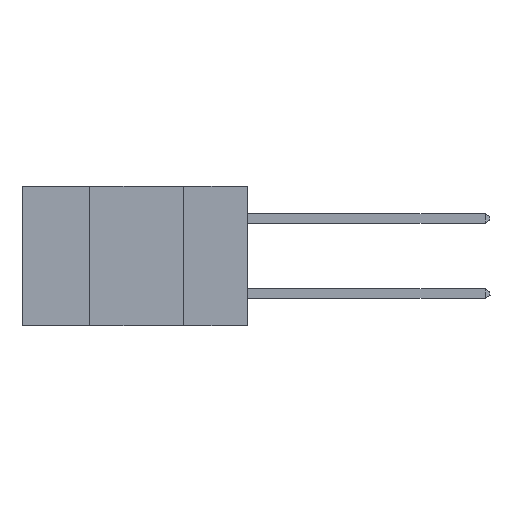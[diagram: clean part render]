
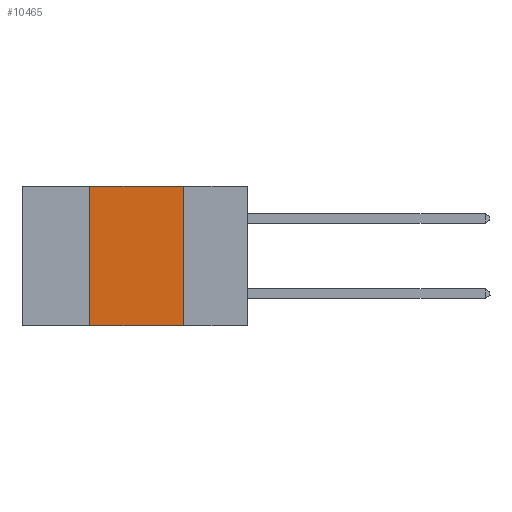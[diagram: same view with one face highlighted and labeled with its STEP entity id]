
A CAD part, left-side view. The second image highlights one B-rep face of the part: STEP entity #10465.
In plain terms, the highlighted planar face has unit normal (-1, 0, 0).
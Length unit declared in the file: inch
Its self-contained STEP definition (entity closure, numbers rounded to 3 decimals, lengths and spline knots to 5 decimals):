
#388 = EDGE_CURVE ( 'NONE', #13627, #13392, #3850, .T. ) ;
#574 = FACE_OUTER_BOUND ( 'NONE', #3345, .T. ) ;
#720 = CARTESIAN_POINT ( 'NONE',  ( 0., 0.6, -0.37 ) ) ;
#824 = AXIS2_PLACEMENT_3D ( 'NONE', #9727, #4533, #14275 ) ;
#936 = ORIENTED_EDGE ( 'NONE', *, *, #12613, .F. ) ;
#942 = VECTOR ( 'NONE', #10215, 39.37008 ) ;
#1697 = PLANE ( 'NONE',  #824 ) ;
#1739 = VECTOR ( 'NONE', #6484, 39.37008 ) ;
#1823 = DIRECTION ( 'NONE',  ( 0., -1., 0. ) ) ;
#3214 = CARTESIAN_POINT ( 'NONE',  ( 0., 0.42, 0. ) ) ;
#3345 = EDGE_LOOP ( 'NONE', ( #936, #15327, #5585, #11309 ) ) ;
#3572 = DIRECTION ( 'NONE',  ( 0., 0., 1. ) ) ;
#3850 = LINE ( 'NONE', #5134, #1739 ) ;
#4533 = DIRECTION ( 'NONE',  ( 1., 0., 0. ) ) ;
#5134 = CARTESIAN_POINT ( 'NONE',  ( 0., 0.6, 0. ) ) ;
#5585 = ORIENTED_EDGE ( 'NONE', *, *, #8709, .F. ) ;
#6321 = CARTESIAN_POINT ( 'NONE',  ( 0., 0.17, 0. ) ) ;
#6484 = DIRECTION ( 'NONE',  ( 0., -1., 0. ) ) ;
#6629 = LINE ( 'NONE', #3214, #14328 ) ;
#7680 = CARTESIAN_POINT ( 'NONE',  ( 0., 0.17, -0.37 ) ) ;
#7715 = CARTESIAN_POINT ( 'NONE',  ( 0., 0.17, 0. ) ) ;
#8709 = EDGE_CURVE ( 'NONE', #11583, #13627, #6629, .T. ) ;
#8852 = VECTOR ( 'NONE', #1823, 39.37008 ) ;
#9145 = CARTESIAN_POINT ( 'NONE',  ( 0., 0.42, 0. ) ) ;
#9727 = CARTESIAN_POINT ( 'NONE',  ( 0., 0.6, 0. ) ) ;
#10215 = DIRECTION ( 'NONE',  ( 0., 0., -1. ) ) ;
#10465 = ADVANCED_FACE ( 'NONE', ( #574 ), #1697, .F. ) ;
#11309 = ORIENTED_EDGE ( 'NONE', *, *, #12347, .T. ) ;
#11376 = CARTESIAN_POINT ( 'NONE',  ( 0., 0.42, -0.37 ) ) ;
#11583 = VERTEX_POINT ( 'NONE', #11376 ) ;
#12347 = EDGE_CURVE ( 'NONE', #11583, #13204, #13130, .T. ) ;
#12613 = EDGE_CURVE ( 'NONE', #13392, #13204, #14644, .T. ) ;
#13130 = LINE ( 'NONE', #720, #8852 ) ;
#13204 = VERTEX_POINT ( 'NONE', #7680 ) ;
#13392 = VERTEX_POINT ( 'NONE', #6321 ) ;
#13627 = VERTEX_POINT ( 'NONE', #9145 ) ;
#14275 = DIRECTION ( 'NONE',  ( 0., 0., -1. ) ) ;
#14328 = VECTOR ( 'NONE', #3572, 39.37008 ) ;
#14644 = LINE ( 'NONE', #7715, #942 ) ;
#15327 = ORIENTED_EDGE ( 'NONE', *, *, #388, .F. ) ;
